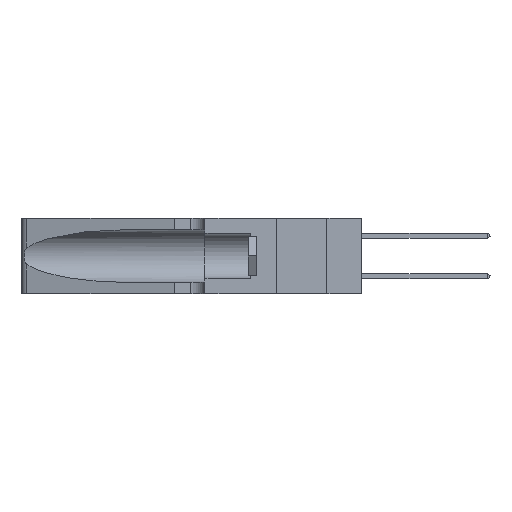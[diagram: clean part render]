
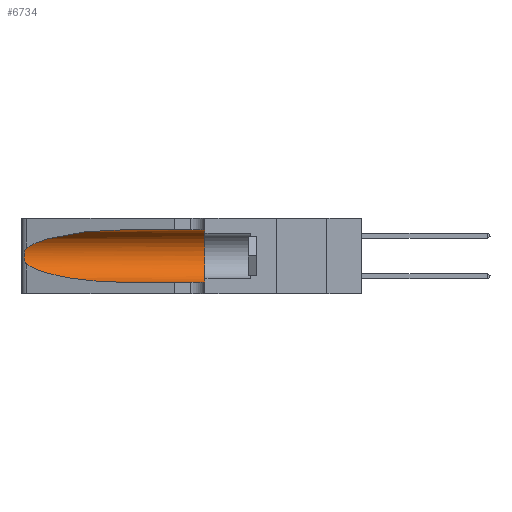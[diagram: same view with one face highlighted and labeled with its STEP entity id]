
A CAD part, left-side view. The second image highlights one B-rep face of the part: STEP entity #6734.
In plain terms, the highlighted cylindrical face has radius 3.308 mm (diameter 6.617 mm), a partial arc.
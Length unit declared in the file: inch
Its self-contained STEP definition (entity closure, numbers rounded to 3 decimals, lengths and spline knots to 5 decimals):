
#82 = CARTESIAN_POINT ( 'NONE',  ( 0.25854, 1.2359, 0.20912 ) ) ;
#243 = ORIENTED_EDGE ( 'NONE', *, *, #27306, .T. ) ;
#603 = ORIENTED_EDGE ( 'NONE', *, *, #8618, .F. ) ;
#2476 =( BOUNDED_CURVE ( )  B_SPLINE_CURVE ( 3, ( #11412, #32103, #14441, #35065 ),
 .UNSPECIFIED., .F., .T. ) 
 B_SPLINE_CURVE_WITH_KNOTS ( ( 4, 4 ),
 ( 3.44316, 4.71239 ),
 .UNSPECIFIED. ) 
 CURVE ( )  GEOMETRIC_REPRESENTATION_ITEM ( )  RATIONAL_B_SPLINE_CURVE ( ( 1., 0.87, 0.87, 1. ) ) 
 REPRESENTATION_ITEM ( '' )  );
#2653 = EDGE_CURVE ( 'NONE', #27196, #17999, #37612, .T. ) ;
#3090 = CARTESIAN_POINT ( 'NONE',  ( 0.26075, 1.23896, 0.19203 ) ) ;
#3730 = DIRECTION ( 'NONE',  ( 0., -1., 0. ) ) ;
#4740 = VERTEX_POINT ( 'NONE', #16687 ) ;
#6083 = DIRECTION ( 'NONE',  ( 0., -1., 0. ) ) ;
#6130 = CARTESIAN_POINT ( 'NONE',  ( 0.26017, 1.23833, 0.17102 ) ) ;
#6734 = ADVANCED_FACE ( 'NONE', ( #34814 ), #21031, .F. ) ;
#7888 = EDGE_LOOP ( 'NONE', ( #16537, #243, #36409, #25540, #603, #33634 ) ) ;
#8508 = CARTESIAN_POINT ( 'NONE',  ( 0.1305, 0.35, 0.05475 ) ) ;
#8618 = EDGE_CURVE ( 'NONE', #17999, #33026, #33748, .T. ) ;
#9201 = CARTESIAN_POINT ( 'NONE',  ( 0.25789, 1.23486, 0.15765 ) ) ;
#10752 = EDGE_CURVE ( 'NONE', #4740, #36997, #2476, .T. ) ;
#11003 = VECTOR ( 'NONE', #3730, 39.37008 ) ;
#11412 = CARTESIAN_POINT ( 'NONE',  ( 0.25487, 1.22718, 0.14631 ) ) ;
#12207 = CARTESIAN_POINT ( 'NONE',  ( 0.25555, 1.22993, 0.14849 ) ) ;
#12312 = EDGE_CURVE ( 'NONE', #36997, #33026, #32739, .T. ) ;
#12378 = CARTESIAN_POINT ( 'NONE',  ( 0.1305, 0.72297, 0.31525 ) ) ;
#12877 = CARTESIAN_POINT ( 'NONE',  ( 0.1305, 1.61858, 0.05475 ) ) ;
#14441 = CARTESIAN_POINT ( 'NONE',  ( 0.18966, 0.96281, 0.05475 ) ) ;
#15114 = CARTESIAN_POINT ( 'NONE',  ( 0.25555, 1.22994, 0.2215 ) ) ;
#16537 = ORIENTED_EDGE ( 'NONE', *, *, #28254, .T. ) ;
#16619 = CARTESIAN_POINT ( 'NONE',  ( 0.1305, 0.72297, 0.05475 ) ) ;
#16645 = AXIS2_PLACEMENT_3D ( 'NONE', #34879, #17234, #37859 ) ;
#16687 = CARTESIAN_POINT ( 'NONE',  ( 0.25487, 1.22718, 0.14631 ) ) ;
#17234 = DIRECTION ( 'NONE',  ( 0., 1., 0. ) ) ;
#17999 = VERTEX_POINT ( 'NONE', #32551 ) ;
#18118 = CARTESIAN_POINT ( 'NONE',  ( 0.25787, 1.23484, 0.2124 ) ) ;
#18530 = CARTESIAN_POINT ( 'NONE',  ( 0.25487, 1.22718, 0.22369 ) ) ;
#21031 = CYLINDRICAL_SURFACE ( 'NONE', #32436, 0.13025 ) ;
#21107 = CARTESIAN_POINT ( 'NONE',  ( 0.26018, 1.23835, 0.19895 ) ) ;
#22906 = VECTOR ( 'NONE', #6083, 39.37008 ) ;
#24083 = CARTESIAN_POINT ( 'NONE',  ( 0.26075, 1.23896, 0.178 ) ) ;
#25540 = ORIENTED_EDGE ( 'NONE', *, *, #12312, .T. ) ;
#25740 = VERTEX_POINT ( 'NONE', #37265 ) ;
#25759 = DIRECTION ( 'NONE',  ( 0., -1., 0. ) ) ;
#26972 = CARTESIAN_POINT ( 'NONE',  ( 0.1305, 1.61858, 0.31525 ) ) ;
#27027 = CARTESIAN_POINT ( 'NONE',  ( 0.25856, 1.23593, 0.16098 ) ) ;
#27196 = VERTEX_POINT ( 'NONE', #29335 ) ;
#27306 = EDGE_CURVE ( 'NONE', #25740, #4740, #37713, .T. ) ;
#28254 = EDGE_CURVE ( 'NONE', #27196, #25740, #31579, .T. ) ;
#28699 = CARTESIAN_POINT ( 'NONE',  ( 0.1305, 1.61858, 0.185 ) ) ;
#29335 = CARTESIAN_POINT ( 'NONE',  ( 0.1305, 0.72297, 0.31525 ) ) ;
#29811 = CARTESIAN_POINT ( 'NONE',  ( 0.25487, 1.22718, 0.22369 ) ) ;
#29950 = CARTESIAN_POINT ( 'NONE',  ( 0.25639, 1.23186, 0.15144 ) ) ;
#31579 =( BOUNDED_CURVE ( )  B_SPLINE_CURVE ( 3, ( #12378, #33181, #36144, #18530 ),
 .UNSPECIFIED., .F., .T. ) 
 B_SPLINE_CURVE_WITH_KNOTS ( ( 4, 4 ),
 ( 1.5708, 2.84003 ),
 .UNSPECIFIED. ) 
 CURVE ( )  GEOMETRIC_REPRESENTATION_ITEM ( )  RATIONAL_B_SPLINE_CURVE ( ( 1., 0.87, 0.87, 1. ) ) 
 REPRESENTATION_ITEM ( '' )  );
#31623 = DIRECTION ( 'NONE',  ( 0., 0., -1. ) ) ;
#32103 = CARTESIAN_POINT ( 'NONE',  ( 0.2373, 1.15595, 0.08982 ) ) ;
#32436 = AXIS2_PLACEMENT_3D ( 'NONE', #28699, #25759, #31623 ) ;
#32551 = CARTESIAN_POINT ( 'NONE',  ( 0.1305, 0.35, 0.31525 ) ) ;
#32739 = LINE ( 'NONE', #12877, #11003 ) ;
#32914 = CARTESIAN_POINT ( 'NONE',  ( 0.25487, 1.22718, 0.14631 ) ) ;
#33026 = VERTEX_POINT ( 'NONE', #8508 ) ;
#33181 = CARTESIAN_POINT ( 'NONE',  ( 0.18966, 0.96281, 0.31525 ) ) ;
#33634 = ORIENTED_EDGE ( 'NONE', *, *, #2653, .F. ) ;
#33748 = CIRCLE ( 'NONE', #16645, 0.13025 ) ;
#34814 = FACE_OUTER_BOUND ( 'NONE', #7888, .T. ) ;
#34879 = CARTESIAN_POINT ( 'NONE',  ( 0.1305, 0.35, 0.185 ) ) ;
#35065 = CARTESIAN_POINT ( 'NONE',  ( 0.1305, 0.72297, 0.05475 ) ) ;
#35733 = CARTESIAN_POINT ( 'NONE',  ( 0.25639, 1.23184, 0.21858 ) ) ;
#36144 = CARTESIAN_POINT ( 'NONE',  ( 0.2373, 1.15595, 0.28018 ) ) ;
#36409 = ORIENTED_EDGE ( 'NONE', *, *, #10752, .T. ) ;
#36997 = VERTEX_POINT ( 'NONE', #16619 ) ;
#37265 = CARTESIAN_POINT ( 'NONE',  ( 0.25487, 1.22718, 0.22369 ) ) ;
#37612 = LINE ( 'NONE', #26972, #22906 ) ;
#37713 = B_SPLINE_CURVE_WITH_KNOTS ( 'NONE', 3,
 ( #29811, #15114, #35733, #18118, #82, #21107, #3090, #24083, #6130, #27027, #9201, #29950, #12207, #32914 ),
 .UNSPECIFIED., .F., .F.,
 ( 4, 2, 2, 2, 2, 2, 4 ),
 ( 0., 0.00027, 0.00053, 0.00107, 0.0016, 0.00187, 0.00214 ),
 .UNSPECIFIED. ) ;
#37859 = DIRECTION ( 'NONE',  ( 0., 0., 1. ) ) ;
